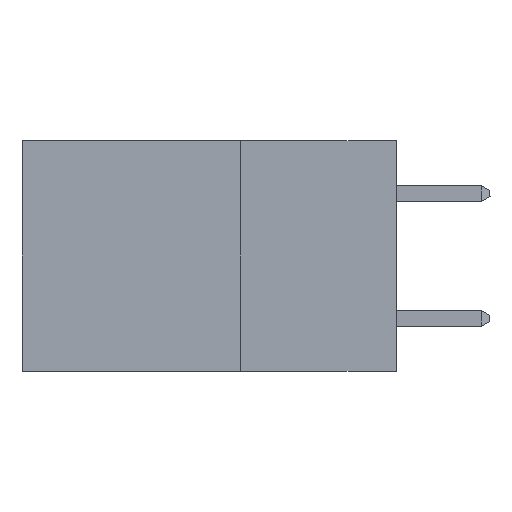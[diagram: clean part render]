
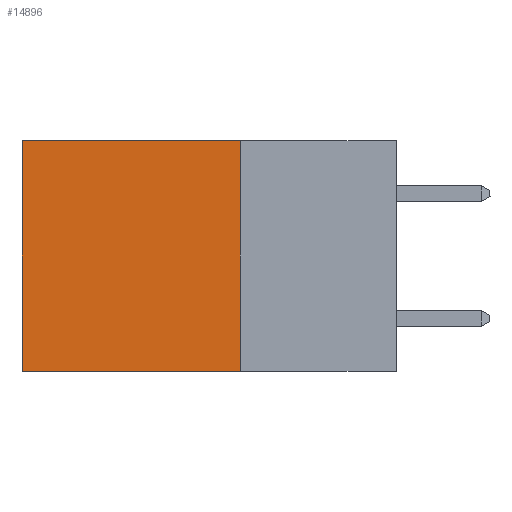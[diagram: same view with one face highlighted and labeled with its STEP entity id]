
A CAD part, left-side view. The second image highlights one B-rep face of the part: STEP entity #14896.
In plain terms, the highlighted planar face has unit normal (-1, 0, 0).
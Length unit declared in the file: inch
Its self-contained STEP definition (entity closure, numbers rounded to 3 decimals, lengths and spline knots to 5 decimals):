
#854 = VECTOR ( 'NONE', #5771, 39.37008 ) ;
#1310 = PLANE ( 'NONE',  #5077 ) ;
#1519 = LINE ( 'NONE', #15886, #18131 ) ;
#2958 = VERTEX_POINT ( 'NONE', #5653 ) ;
#3153 = CARTESIAN_POINT ( 'NONE',  ( 0.298, 0.25, -0.37 ) ) ;
#4511 = EDGE_CURVE ( 'NONE', #14485, #5509, #7862, .T. ) ;
#4801 = DIRECTION ( 'NONE',  ( 0., 0., -1. ) ) ;
#5077 = AXIS2_PLACEMENT_3D ( 'NONE', #12576, #7587, #7661 ) ;
#5292 = EDGE_LOOP ( 'NONE', ( #5552, #11229, #19917, #10453 ) ) ;
#5368 = CARTESIAN_POINT ( 'NONE',  ( 0.298, 0.25, 0. ) ) ;
#5509 = VERTEX_POINT ( 'NONE', #15235 ) ;
#5552 = ORIENTED_EDGE ( 'NONE', *, *, #7003, .T. ) ;
#5653 = CARTESIAN_POINT ( 'NONE',  ( 0.298, 0.6, 0. ) ) ;
#5771 = DIRECTION ( 'NONE',  ( 0., 1., 0. ) ) ;
#6050 = CARTESIAN_POINT ( 'NONE',  ( 0.298, 0.25, 0. ) ) ;
#7003 = EDGE_CURVE ( 'NONE', #2958, #5509, #1519, .T. ) ;
#7148 = FACE_OUTER_BOUND ( 'NONE', #5292, .T. ) ;
#7587 = DIRECTION ( 'NONE',  ( 1., 0., 0. ) ) ;
#7661 = DIRECTION ( 'NONE',  ( 0., 0., -1. ) ) ;
#7862 = LINE ( 'NONE', #12241, #854 ) ;
#8796 = VERTEX_POINT ( 'NONE', #5368 ) ;
#10277 = VECTOR ( 'NONE', #18834, 39.37008 ) ;
#10453 = ORIENTED_EDGE ( 'NONE', *, *, #14273, .T. ) ;
#11229 = ORIENTED_EDGE ( 'NONE', *, *, #4511, .F. ) ;
#11764 = VECTOR ( 'NONE', #16964, 39.37008 ) ;
#12241 = CARTESIAN_POINT ( 'NONE',  ( 0.298, 0.25, -0.37 ) ) ;
#12576 = CARTESIAN_POINT ( 'NONE',  ( 0.298, 0.25, 0. ) ) ;
#13604 = CARTESIAN_POINT ( 'NONE',  ( 0.298, 0.25, 0. ) ) ;
#14273 = EDGE_CURVE ( 'NONE', #8796, #2958, #19840, .T. ) ;
#14485 = VERTEX_POINT ( 'NONE', #3153 ) ;
#14896 = ADVANCED_FACE ( 'NONE', ( #7148 ), #1310, .F. ) ;
#15235 = CARTESIAN_POINT ( 'NONE',  ( 0.298, 0.6, -0.37 ) ) ;
#15886 = CARTESIAN_POINT ( 'NONE',  ( 0.298, 0.6, 0. ) ) ;
#16964 = DIRECTION ( 'NONE',  ( 0., 1., 0. ) ) ;
#18131 = VECTOR ( 'NONE', #4801, 39.37008 ) ;
#18634 = EDGE_CURVE ( 'NONE', #8796, #14485, #19373, .T. ) ;
#18834 = DIRECTION ( 'NONE',  ( 0., 0., -1. ) ) ;
#19373 = LINE ( 'NONE', #6050, #10277 ) ;
#19840 = LINE ( 'NONE', #13604, #11764 ) ;
#19917 = ORIENTED_EDGE ( 'NONE', *, *, #18634, .F. ) ;
